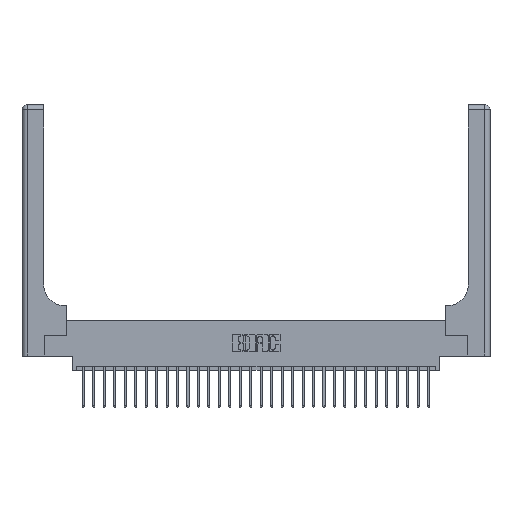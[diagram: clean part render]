
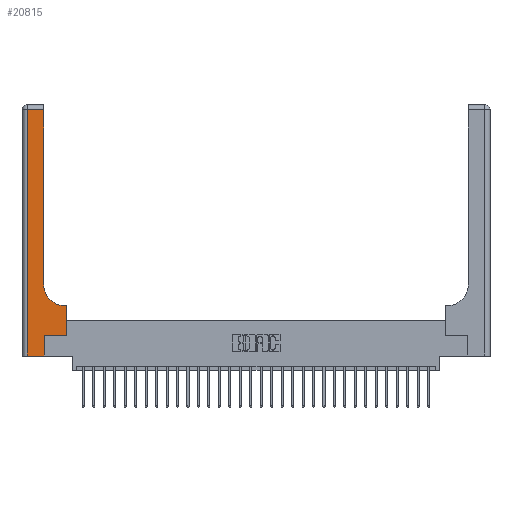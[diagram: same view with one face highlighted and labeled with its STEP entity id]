
A CAD part, top view. The second image highlights one B-rep face of the part: STEP entity #20815.
In plain terms, the highlighted planar face has unit normal (0, 0, 1).
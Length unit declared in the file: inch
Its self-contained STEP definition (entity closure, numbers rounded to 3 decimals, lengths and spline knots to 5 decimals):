
#278 = DIRECTION ( 'NONE',  ( 0., -1., 0. ) ) ;
#1083 = DIRECTION ( 'NONE',  ( 1., 0., 0. ) ) ;
#1362 = EDGE_CURVE ( 'NONE', #22494, #27047, #27820, .T. ) ;
#1369 = VECTOR ( 'NONE', #22761, 39.37008 ) ;
#1390 = DIRECTION ( 'NONE',  ( 0., 0., -1. ) ) ;
#1863 = LINE ( 'NONE', #28754, #7613 ) ;
#2231 = VECTOR ( 'NONE', #9646, 39.37008 ) ;
#2877 = LINE ( 'NONE', #15954, #2231 ) ;
#3142 = CARTESIAN_POINT ( 'NONE',  ( 0.528, 0.25, 0.37 ) ) ;
#3593 = FACE_OUTER_BOUND ( 'NONE', #28146, .T. ) ;
#3600 = CARTESIAN_POINT ( 'NONE',  ( 0.528, 0.6, 0.37 ) ) ;
#4926 = ORIENTED_EDGE ( 'NONE', *, *, #24070, .T. ) ;
#5107 = ORIENTED_EDGE ( 'NONE', *, *, #1362, .T. ) ;
#5328 = EDGE_CURVE ( 'NONE', #7800, #15353, #15982, .T. ) ;
#6208 = VECTOR ( 'NONE', #278, 39.37008 ) ;
#7176 = VERTEX_POINT ( 'NONE', #3600 ) ;
#7613 = VECTOR ( 'NONE', #17560, 39.37008 ) ;
#7800 = VERTEX_POINT ( 'NONE', #8563 ) ;
#7880 = EDGE_CURVE ( 'NONE', #14354, #26308, #22483, .T. ) ;
#8013 = CIRCLE ( 'NONE', #13169, 0.25 ) ;
#8247 = DIRECTION ( 'NONE',  ( 1., 0., 0. ) ) ;
#8563 = CARTESIAN_POINT ( 'NONE',  ( 0.06, 2.94, 0.37 ) ) ;
#8637 = ORIENTED_EDGE ( 'NONE', *, *, #14625, .T. ) ;
#9058 = EDGE_CURVE ( 'NONE', #15353, #22494, #27543, .T. ) ;
#9478 = CARTESIAN_POINT ( 'NONE',  ( 0.26, 0.85, 0.37 ) ) ;
#9646 = DIRECTION ( 'NONE',  ( 1., 0., 0. ) ) ;
#10245 = VECTOR ( 'NONE', #14434, 39.37008 ) ;
#10305 = DIRECTION ( 'NONE',  ( 0., 0., -1. ) ) ;
#10657 = DIRECTION ( 'NONE',  ( -1., 0., 0. ) ) ;
#11780 = CARTESIAN_POINT ( 'NONE',  ( 0.26, 3., 0.37 ) ) ;
#12114 = DIRECTION ( 'NONE',  ( 0., 1., 0. ) ) ;
#12557 = CARTESIAN_POINT ( 'NONE',  ( 0., 3., 0.37 ) ) ;
#12993 = CARTESIAN_POINT ( 'NONE',  ( 0., 2.94, 0.37 ) ) ;
#13169 = AXIS2_PLACEMENT_3D ( 'NONE', #26003, #10305, #8247 ) ;
#13953 = ORIENTED_EDGE ( 'NONE', *, *, #25807, .T. ) ;
#14296 = VECTOR ( 'NONE', #12114, 39.37008 ) ;
#14354 = VERTEX_POINT ( 'NONE', #9478 ) ;
#14434 = DIRECTION ( 'NONE',  ( 0., 1., 0. ) ) ;
#14625 = EDGE_CURVE ( 'NONE', #18458, #7176, #23245, .T. ) ;
#14785 = ORIENTED_EDGE ( 'NONE', *, *, #20922, .T. ) ;
#15353 = VERTEX_POINT ( 'NONE', #15432 ) ;
#15432 = CARTESIAN_POINT ( 'NONE',  ( 0.06, 0., 0.37 ) ) ;
#15954 = CARTESIAN_POINT ( 'NONE',  ( 0.265, 0.25, 0.37 ) ) ;
#15982 = LINE ( 'NONE', #25383, #6208 ) ;
#16044 = ORIENTED_EDGE ( 'NONE', *, *, #5328, .T. ) ;
#16074 = ORIENTED_EDGE ( 'NONE', *, *, #7880, .T. ) ;
#16797 = AXIS2_PLACEMENT_3D ( 'NONE', #12557, #1390, #21513 ) ;
#16945 = VERTEX_POINT ( 'NONE', #22017 ) ;
#16952 = ORIENTED_EDGE ( 'NONE', *, *, #18788, .T. ) ;
#17150 = CARTESIAN_POINT ( 'NONE',  ( 0.528, 0.25, 0.37 ) ) ;
#17410 = ORIENTED_EDGE ( 'NONE', *, *, #9058, .T. ) ;
#17560 = DIRECTION ( 'NONE',  ( -1., 0., 0. ) ) ;
#17670 = CARTESIAN_POINT ( 'NONE',  ( 0.26, 2.94, 0.37 ) ) ;
#18458 = VERTEX_POINT ( 'NONE', #17150 ) ;
#18788 = EDGE_CURVE ( 'NONE', #27047, #18458, #2877, .T. ) ;
#20203 = VECTOR ( 'NONE', #1083, 39.37008 ) ;
#20815 = ADVANCED_FACE ( 'NONE', ( #3593 ), #23695, .F. ) ;
#20922 = EDGE_CURVE ( 'NONE', #26308, #7800, #21796, .T. ) ;
#21239 = CARTESIAN_POINT ( 'NONE',  ( 0.265, 0.25, 0.37 ) ) ;
#21513 = DIRECTION ( 'NONE',  ( -1., 0., 0. ) ) ;
#21796 = LINE ( 'NONE', #12993, #27122 ) ;
#22017 = CARTESIAN_POINT ( 'NONE',  ( 0.51, 0.6, 0.37 ) ) ;
#22483 = LINE ( 'NONE', #11780, #1369 ) ;
#22494 = VERTEX_POINT ( 'NONE', #23665 ) ;
#22761 = DIRECTION ( 'NONE',  ( 0., 1., 0. ) ) ;
#23245 = LINE ( 'NONE', #3142, #14296 ) ;
#23665 = CARTESIAN_POINT ( 'NONE',  ( 0.265, 0., 0.37 ) ) ;
#23695 = PLANE ( 'NONE',  #16797 ) ;
#24070 = EDGE_CURVE ( 'NONE', #16945, #14354, #8013, .T. ) ;
#25383 = CARTESIAN_POINT ( 'NONE',  ( 0.06, 3., 0.37 ) ) ;
#25602 = CARTESIAN_POINT ( 'NONE',  ( 0.265, 0., 0.37 ) ) ;
#25760 = CARTESIAN_POINT ( 'NONE',  ( 0., 0., 0.37 ) ) ;
#25807 = EDGE_CURVE ( 'NONE', #7176, #16945, #1863, .T. ) ;
#26003 = CARTESIAN_POINT ( 'NONE',  ( 0.51, 0.85, 0.37 ) ) ;
#26308 = VERTEX_POINT ( 'NONE', #17670 ) ;
#27047 = VERTEX_POINT ( 'NONE', #21239 ) ;
#27122 = VECTOR ( 'NONE', #10657, 39.37008 ) ;
#27543 = LINE ( 'NONE', #25760, #20203 ) ;
#27820 = LINE ( 'NONE', #25602, #10245 ) ;
#28146 = EDGE_LOOP ( 'NONE', ( #16074, #14785, #16044, #17410, #5107, #16952, #8637, #13953, #4926 ) ) ;
#28754 = CARTESIAN_POINT ( 'NONE',  ( 0.26, 0.6, 0.37 ) ) ;
